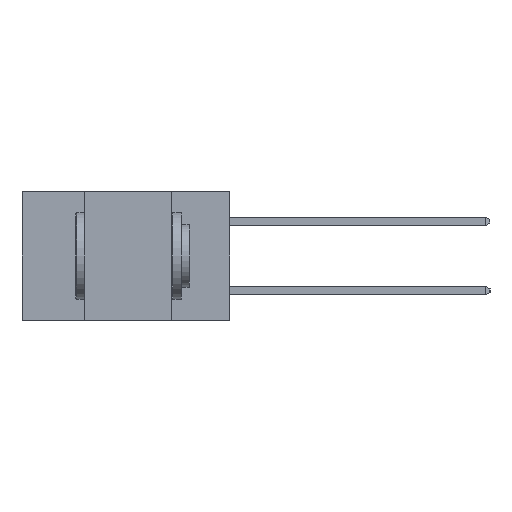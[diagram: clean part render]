
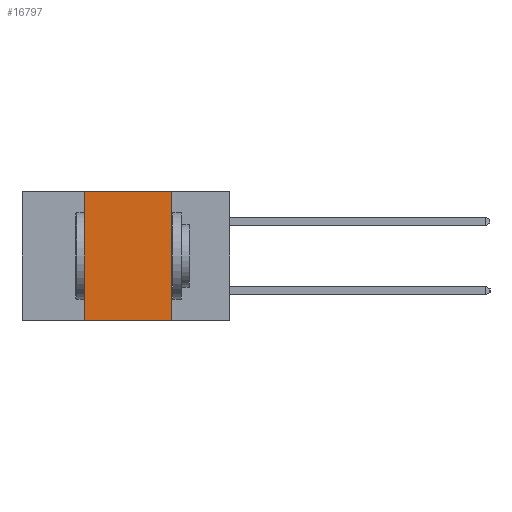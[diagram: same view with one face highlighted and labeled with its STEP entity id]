
A CAD part, left-side view. The second image highlights one B-rep face of the part: STEP entity #16797.
In plain terms, the highlighted planar face has unit normal (-1, 0, 0).
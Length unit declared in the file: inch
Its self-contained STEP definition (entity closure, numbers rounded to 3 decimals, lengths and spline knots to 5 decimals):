
#416 = DIRECTION ( 'NONE',  ( 0., 0., -1. ) ) ;
#716 = PLANE ( 'NONE',  #18906 ) ;
#2626 = CARTESIAN_POINT ( 'NONE',  ( 0., 0.42, 0. ) ) ;
#2646 = DIRECTION ( 'NONE',  ( 1., 0., 0. ) ) ;
#2945 = LINE ( 'NONE', #17587, #22702 ) ;
#3115 = EDGE_CURVE ( 'NONE', #8294, #4985, #6715, .T. ) ;
#3681 = EDGE_LOOP ( 'NONE', ( #5743, #8166, #6069, #4543 ) ) ;
#4099 = EDGE_CURVE ( 'NONE', #16461, #8294, #15014, .T. ) ;
#4543 = ORIENTED_EDGE ( 'NONE', *, *, #16723, .T. ) ;
#4665 = CARTESIAN_POINT ( 'NONE',  ( 0., 0.17, -0.37 ) ) ;
#4822 = VECTOR ( 'NONE', #8065, 39.37008 ) ;
#4985 = VERTEX_POINT ( 'NONE', #10703 ) ;
#5472 = CARTESIAN_POINT ( 'NONE',  ( 0., 0.42, -0.37 ) ) ;
#5743 = ORIENTED_EDGE ( 'NONE', *, *, #12471, .F. ) ;
#6069 = ORIENTED_EDGE ( 'NONE', *, *, #4099, .F. ) ;
#6715 = LINE ( 'NONE', #20090, #11784 ) ;
#7497 = CARTESIAN_POINT ( 'NONE',  ( 0., 0.42, -0.37 ) ) ;
#7691 = FACE_OUTER_BOUND ( 'NONE', #3681, .T. ) ;
#8065 = DIRECTION ( 'NONE',  ( 0., 0., 1. ) ) ;
#8166 = ORIENTED_EDGE ( 'NONE', *, *, #3115, .F. ) ;
#8294 = VERTEX_POINT ( 'NONE', #2626 ) ;
#8349 = VERTEX_POINT ( 'NONE', #4665 ) ;
#9466 = LINE ( 'NONE', #23401, #18990 ) ;
#10703 = CARTESIAN_POINT ( 'NONE',  ( 0., 0.17, 0. ) ) ;
#11784 = VECTOR ( 'NONE', #20058, 39.37008 ) ;
#12471 = EDGE_CURVE ( 'NONE', #4985, #8349, #2945, .T. ) ;
#14152 = CARTESIAN_POINT ( 'NONE',  ( 0., 0.6, 0. ) ) ;
#15014 = LINE ( 'NONE', #7497, #4822 ) ;
#15736 = DIRECTION ( 'NONE',  ( 0., -1., 0. ) ) ;
#16053 = DIRECTION ( 'NONE',  ( 0., 0., -1. ) ) ;
#16461 = VERTEX_POINT ( 'NONE', #5472 ) ;
#16723 = EDGE_CURVE ( 'NONE', #16461, #8349, #9466, .T. ) ;
#16797 = ADVANCED_FACE ( 'NONE', ( #7691 ), #716, .F. ) ;
#17587 = CARTESIAN_POINT ( 'NONE',  ( 0., 0.17, -0.37 ) ) ;
#18906 = AXIS2_PLACEMENT_3D ( 'NONE', #14152, #2646, #16053 ) ;
#18990 = VECTOR ( 'NONE', #15736, 39.37008 ) ;
#20058 = DIRECTION ( 'NONE',  ( 0., -1., 0. ) ) ;
#20090 = CARTESIAN_POINT ( 'NONE',  ( 0., 0.6, 0. ) ) ;
#22702 = VECTOR ( 'NONE', #416, 39.37008 ) ;
#23401 = CARTESIAN_POINT ( 'NONE',  ( 0., 0.6, -0.37 ) ) ;
